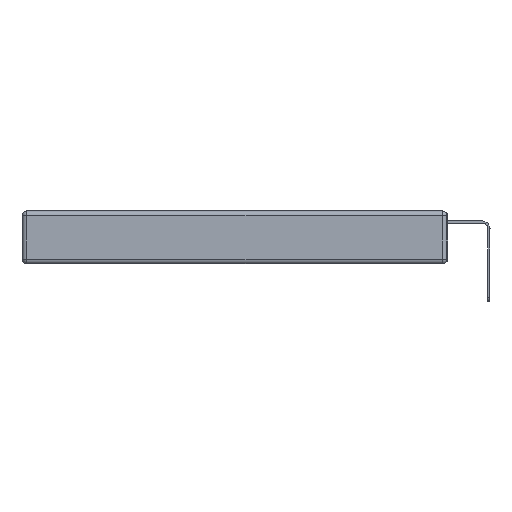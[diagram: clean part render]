
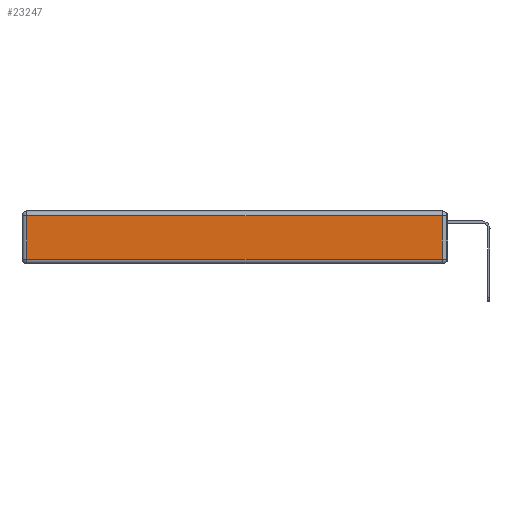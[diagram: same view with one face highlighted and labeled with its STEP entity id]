
A CAD part, left-side view. The second image highlights one B-rep face of the part: STEP entity #23247.
In plain terms, the highlighted planar face has unit normal (-1, 0, 0).
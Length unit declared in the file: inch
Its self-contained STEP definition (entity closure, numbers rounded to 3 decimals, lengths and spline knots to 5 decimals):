
#9 = CARTESIAN_POINT ( 'NONE',  ( 0., 2.72, -0.03 ) ) ;
#646 = VECTOR ( 'NONE', #25265, 39.37008 ) ;
#1935 = PLANE ( 'NONE',  #17522 ) ;
#2212 = CARTESIAN_POINT ( 'NONE',  ( 0., 0., -0.313 ) ) ;
#2584 = VECTOR ( 'NONE', #6066, 39.37008 ) ;
#2819 = ORIENTED_EDGE ( 'NONE', *, *, #20467, .T. ) ;
#4353 = EDGE_CURVE ( 'NONE', #24543, #6507, #25269, .T. ) ;
#4540 = VECTOR ( 'NONE', #24804, 39.37008 ) ;
#6066 = DIRECTION ( 'NONE',  ( 0., 1., 0. ) ) ;
#6507 = VERTEX_POINT ( 'NONE', #11959 ) ;
#8178 = DIRECTION ( 'NONE',  ( 0., 0., 1. ) ) ;
#8205 = CARTESIAN_POINT ( 'NONE',  ( 0., 2.75, -0.03 ) ) ;
#8745 = EDGE_CURVE ( 'NONE', #9628, #24543, #24534, .T. ) ;
#9628 = VERTEX_POINT ( 'NONE', #11269 ) ;
#11269 = CARTESIAN_POINT ( 'NONE',  ( 0., 0.03, -0.03 ) ) ;
#11959 = CARTESIAN_POINT ( 'NONE',  ( 0., 2.72, -0.313 ) ) ;
#12053 = FACE_OUTER_BOUND ( 'NONE', #19346, .T. ) ;
#13387 = LINE ( 'NONE', #19233, #646 ) ;
#13498 = EDGE_CURVE ( 'NONE', #15065, #9628, #13387, .T. ) ;
#13957 = CARTESIAN_POINT ( 'NONE',  ( 0., 0., -0.343 ) ) ;
#15065 = VERTEX_POINT ( 'NONE', #21532 ) ;
#15349 = DIRECTION ( 'NONE',  ( 0., 0., -1. ) ) ;
#16152 = DIRECTION ( 'NONE',  ( -1., 0., 0. ) ) ;
#16602 = LINE ( 'NONE', #2212, #4540 ) ;
#16755 = ORIENTED_EDGE ( 'NONE', *, *, #8745, .T. ) ;
#17522 = AXIS2_PLACEMENT_3D ( 'NONE', #13957, #16152, #8178 ) ;
#19233 = CARTESIAN_POINT ( 'NONE',  ( 0., 0.03, -0.343 ) ) ;
#19346 = EDGE_LOOP ( 'NONE', ( #2819, #22838, #16755, #22811 ) ) ;
#20467 = EDGE_CURVE ( 'NONE', #6507, #15065, #16602, .T. ) ;
#21432 = CARTESIAN_POINT ( 'NONE',  ( 0., 2.72, -0.343 ) ) ;
#21532 = CARTESIAN_POINT ( 'NONE',  ( 0., 0.03, -0.313 ) ) ;
#22811 = ORIENTED_EDGE ( 'NONE', *, *, #4353, .T. ) ;
#22838 = ORIENTED_EDGE ( 'NONE', *, *, #13498, .T. ) ;
#23247 = ADVANCED_FACE ( 'NONE', ( #12053 ), #1935, .T. ) ;
#24534 = LINE ( 'NONE', #8205, #2584 ) ;
#24543 = VERTEX_POINT ( 'NONE', #9 ) ;
#24804 = DIRECTION ( 'NONE',  ( 0., -1., 0. ) ) ;
#25265 = DIRECTION ( 'NONE',  ( 0., 0., 1. ) ) ;
#25269 = LINE ( 'NONE', #21432, #25929 ) ;
#25929 = VECTOR ( 'NONE', #15349, 39.37008 ) ;
